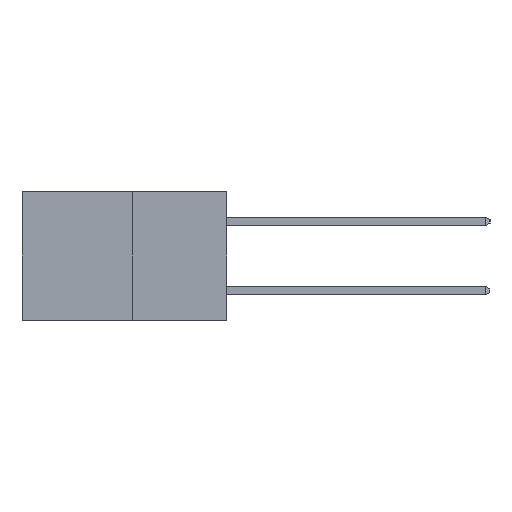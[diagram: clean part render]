
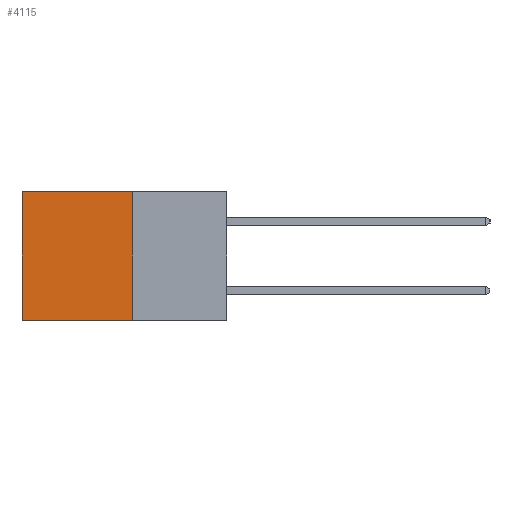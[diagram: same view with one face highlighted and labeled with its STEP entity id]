
A CAD part, left-side view. The second image highlights one B-rep face of the part: STEP entity #4115.
In plain terms, the highlighted planar face has unit normal (-1, 0, 0).
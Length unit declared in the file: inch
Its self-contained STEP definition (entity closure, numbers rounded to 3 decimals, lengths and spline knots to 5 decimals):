
#842 = VECTOR ( 'NONE', #3066, 39.37008 ) ;
#1095 = PLANE ( 'NONE',  #5495 ) ;
#1201 = FACE_OUTER_BOUND ( 'NONE', #7521, .T. ) ;
#1501 = DIRECTION ( 'NONE',  ( 0., 0., -1. ) ) ;
#1638 = LINE ( 'NONE', #4694, #7838 ) ;
#1880 = CARTESIAN_POINT ( 'NONE',  ( 0.277, 0.59, -0.37 ) ) ;
#2021 = DIRECTION ( 'NONE',  ( 0., 0., -1. ) ) ;
#2064 = CARTESIAN_POINT ( 'NONE',  ( 0.277, 0.27, 0. ) ) ;
#2891 = VECTOR ( 'NONE', #8489, 39.37008 ) ;
#3066 = DIRECTION ( 'NONE',  ( 0., 1., 0. ) ) ;
#3071 = CARTESIAN_POINT ( 'NONE',  ( 0.277, 0.27, -0.37 ) ) ;
#4115 = ADVANCED_FACE ( 'NONE', ( #1201 ), #1095, .F. ) ;
#4694 = CARTESIAN_POINT ( 'NONE',  ( 0.277, 0.59, -0.37 ) ) ;
#4815 = ORIENTED_EDGE ( 'NONE', *, *, #7804, .F. ) ;
#5056 = LINE ( 'NONE', #2064, #2891 ) ;
#5211 = EDGE_CURVE ( 'NONE', #8319, #8796, #9619, .T. ) ;
#5280 = VECTOR ( 'NONE', #2021, 39.37008 ) ;
#5311 = CARTESIAN_POINT ( 'NONE',  ( 0.277, 0.27, -0.37 ) ) ;
#5327 = ORIENTED_EDGE ( 'NONE', *, *, #9944, .T. ) ;
#5495 = AXIS2_PLACEMENT_3D ( 'NONE', #5311, #9643, #6240 ) ;
#5706 = EDGE_CURVE ( 'NONE', #6858, #8127, #1638, .T. ) ;
#5797 = ORIENTED_EDGE ( 'NONE', *, *, #5706, .T. ) ;
#5952 = CARTESIAN_POINT ( 'NONE',  ( 0.277, 0.27, -0.37 ) ) ;
#6240 = DIRECTION ( 'NONE',  ( 0., 0., -1. ) ) ;
#6858 = VERTEX_POINT ( 'NONE', #10475 ) ;
#7259 = CARTESIAN_POINT ( 'NONE',  ( 0.277, 0.27, 0. ) ) ;
#7330 = CARTESIAN_POINT ( 'NONE',  ( 0.277, 0.27, -0.37 ) ) ;
#7430 = LINE ( 'NONE', #3071, #842 ) ;
#7521 = EDGE_LOOP ( 'NONE', ( #5797, #4815, #8059, #5327 ) ) ;
#7804 = EDGE_CURVE ( 'NONE', #8796, #8127, #7430, .T. ) ;
#7838 = VECTOR ( 'NONE', #1501, 39.37008 ) ;
#8059 = ORIENTED_EDGE ( 'NONE', *, *, #5211, .F. ) ;
#8127 = VERTEX_POINT ( 'NONE', #1880 ) ;
#8319 = VERTEX_POINT ( 'NONE', #7259 ) ;
#8489 = DIRECTION ( 'NONE',  ( 0., 1., 0. ) ) ;
#8796 = VERTEX_POINT ( 'NONE', #7330 ) ;
#9619 = LINE ( 'NONE', #5952, #5280 ) ;
#9643 = DIRECTION ( 'NONE',  ( 1., 0., 0. ) ) ;
#9944 = EDGE_CURVE ( 'NONE', #8319, #6858, #5056, .T. ) ;
#10475 = CARTESIAN_POINT ( 'NONE',  ( 0.277, 0.59, 0. ) ) ;
